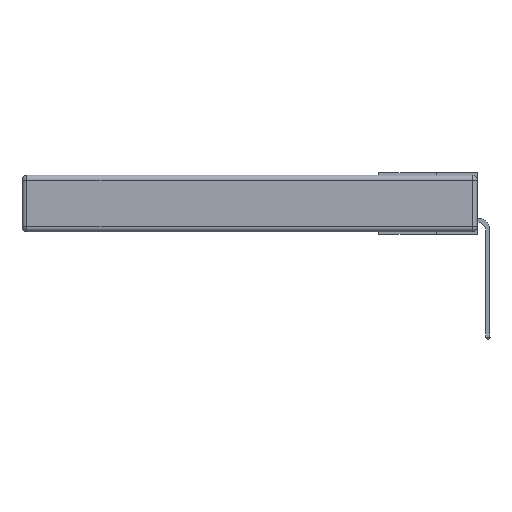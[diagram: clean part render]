
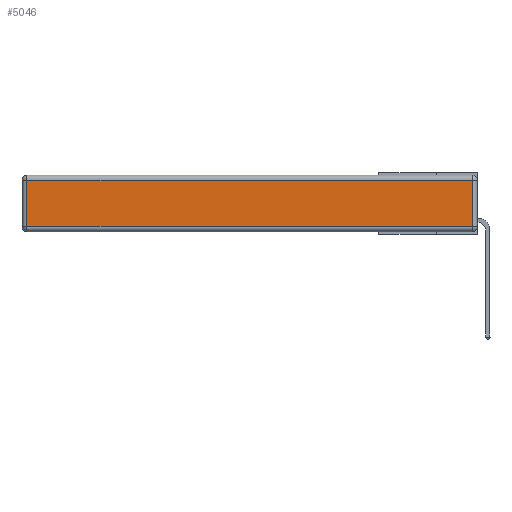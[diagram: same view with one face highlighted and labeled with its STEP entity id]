
A CAD part, left-side view. The second image highlights one B-rep face of the part: STEP entity #5046.
In plain terms, the highlighted planar face has unit normal (-1, 0, 0).
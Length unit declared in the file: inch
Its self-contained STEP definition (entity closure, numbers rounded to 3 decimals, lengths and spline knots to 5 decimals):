
#189 = CARTESIAN_POINT ( 'NONE',  ( 0., 0., -0.313 ) ) ;
#340 = CARTESIAN_POINT ( 'NONE',  ( 0., 2.72, -0.313 ) ) ;
#612 = LINE ( 'NONE', #8824, #8545 ) ;
#614 = VECTOR ( 'NONE', #9989, 39.37008 ) ;
#758 = DIRECTION ( 'NONE',  ( 0., 1., 0. ) ) ;
#1082 = LINE ( 'NONE', #189, #10642 ) ;
#1316 = ORIENTED_EDGE ( 'NONE', *, *, #11085, .T. ) ;
#1380 = LINE ( 'NONE', #9155, #8160 ) ;
#1602 = VERTEX_POINT ( 'NONE', #340 ) ;
#1625 = DIRECTION ( 'NONE',  ( 0., 0., 1. ) ) ;
#2941 = DIRECTION ( 'NONE',  ( -1., 0., 0. ) ) ;
#3031 = DIRECTION ( 'NONE',  ( 0., -1., 0. ) ) ;
#3503 = CARTESIAN_POINT ( 'NONE',  ( 0., 0.03, -0.343 ) ) ;
#3702 = VERTEX_POINT ( 'NONE', #10283 ) ;
#4080 = EDGE_CURVE ( 'NONE', #11478, #1602, #612, .T. ) ;
#4202 = LINE ( 'NONE', #3503, #614 ) ;
#4557 = CARTESIAN_POINT ( 'NONE',  ( 0., 2.72, -0.03 ) ) ;
#4590 = AXIS2_PLACEMENT_3D ( 'NONE', #7561, #2941, #1625 ) ;
#5046 = ADVANCED_FACE ( 'NONE', ( #7827 ), #5515, .T. ) ;
#5515 = PLANE ( 'NONE',  #4590 ) ;
#6046 = ORIENTED_EDGE ( 'NONE', *, *, #4080, .T. ) ;
#6655 = EDGE_CURVE ( 'NONE', #1602, #8313, #1082, .T. ) ;
#7000 = ORIENTED_EDGE ( 'NONE', *, *, #9756, .T. ) ;
#7561 = CARTESIAN_POINT ( 'NONE',  ( 0., 0., -0.343 ) ) ;
#7827 = FACE_OUTER_BOUND ( 'NONE', #10790, .T. ) ;
#8160 = VECTOR ( 'NONE', #758, 39.37008 ) ;
#8313 = VERTEX_POINT ( 'NONE', #11807 ) ;
#8545 = VECTOR ( 'NONE', #8740, 39.37008 ) ;
#8740 = DIRECTION ( 'NONE',  ( 0., 0., -1. ) ) ;
#8824 = CARTESIAN_POINT ( 'NONE',  ( 0., 2.72, -0.343 ) ) ;
#9155 = CARTESIAN_POINT ( 'NONE',  ( 0., 2.75, -0.03 ) ) ;
#9375 = ORIENTED_EDGE ( 'NONE', *, *, #6655, .T. ) ;
#9756 = EDGE_CURVE ( 'NONE', #3702, #11478, #1380, .T. ) ;
#9989 = DIRECTION ( 'NONE',  ( 0., 0., 1. ) ) ;
#10283 = CARTESIAN_POINT ( 'NONE',  ( 0., 0.03, -0.03 ) ) ;
#10642 = VECTOR ( 'NONE', #3031, 39.37008 ) ;
#10790 = EDGE_LOOP ( 'NONE', ( #9375, #1316, #7000, #6046 ) ) ;
#11085 = EDGE_CURVE ( 'NONE', #8313, #3702, #4202, .T. ) ;
#11478 = VERTEX_POINT ( 'NONE', #4557 ) ;
#11807 = CARTESIAN_POINT ( 'NONE',  ( 0., 0.03, -0.313 ) ) ;
